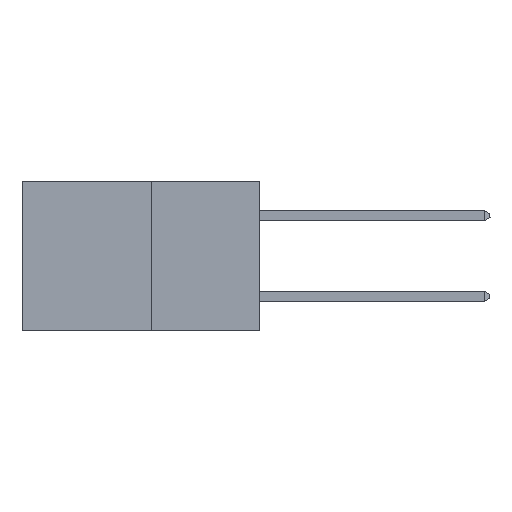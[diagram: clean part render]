
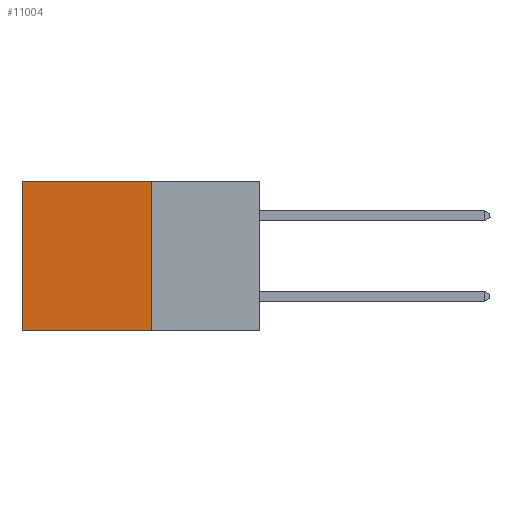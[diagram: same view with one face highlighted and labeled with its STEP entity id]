
A CAD part, left-side view. The second image highlights one B-rep face of the part: STEP entity #11004.
In plain terms, the highlighted planar face has unit normal (-1, 0, 0).
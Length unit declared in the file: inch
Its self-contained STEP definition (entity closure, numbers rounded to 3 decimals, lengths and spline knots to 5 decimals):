
#146 = FACE_OUTER_BOUND ( 'NONE', #1219, .T. ) ;
#1219 = EDGE_LOOP ( 'NONE', ( #10099, #11116, #4568, #2915 ) ) ;
#1784 = DIRECTION ( 'NONE',  ( 0., 1., 0. ) ) ;
#2915 = ORIENTED_EDGE ( 'NONE', *, *, #9272, .T. ) ;
#2984 = LINE ( 'NONE', #14769, #10067 ) ;
#4271 = DIRECTION ( 'NONE',  ( 0., 0., -1. ) ) ;
#4323 = CARTESIAN_POINT ( 'NONE',  ( 0.277, 0.59, -0.37 ) ) ;
#4568 = ORIENTED_EDGE ( 'NONE', *, *, #6917, .F. ) ;
#5737 = EDGE_CURVE ( 'NONE', #11040, #17031, #18094, .T. ) ;
#6049 = CARTESIAN_POINT ( 'NONE',  ( 0.277, 0.59, -0.37 ) ) ;
#6917 = EDGE_CURVE ( 'NONE', #9844, #12047, #13390, .T. ) ;
#6955 = VECTOR ( 'NONE', #4271, 39.37008 ) ;
#8915 = DIRECTION ( 'NONE',  ( 0., 0., -1. ) ) ;
#8993 = CARTESIAN_POINT ( 'NONE',  ( 0.277, 0.27, -0.37 ) ) ;
#9272 = EDGE_CURVE ( 'NONE', #9844, #11040, #13121, .T. ) ;
#9724 = DIRECTION ( 'NONE',  ( 0., 0., -1. ) ) ;
#9748 = VECTOR ( 'NONE', #1784, 39.37008 ) ;
#9844 = VERTEX_POINT ( 'NONE', #9949 ) ;
#9949 = CARTESIAN_POINT ( 'NONE',  ( 0.277, 0.27, 0. ) ) ;
#10067 = VECTOR ( 'NONE', #16122, 39.37008 ) ;
#10099 = ORIENTED_EDGE ( 'NONE', *, *, #5737, .T. ) ;
#10284 = CARTESIAN_POINT ( 'NONE',  ( 0.277, 0.27, 0. ) ) ;
#11004 = ADVANCED_FACE ( 'NONE', ( #146 ), #16634, .F. ) ;
#11040 = VERTEX_POINT ( 'NONE', #11175 ) ;
#11116 = ORIENTED_EDGE ( 'NONE', *, *, #15195, .F. ) ;
#11175 = CARTESIAN_POINT ( 'NONE',  ( 0.277, 0.59, 0. ) ) ;
#11323 = CARTESIAN_POINT ( 'NONE',  ( 0.277, 0.27, -0.37 ) ) ;
#12047 = VERTEX_POINT ( 'NONE', #11323 ) ;
#12934 = VECTOR ( 'NONE', #8915, 39.37008 ) ;
#13121 = LINE ( 'NONE', #10284, #9748 ) ;
#13390 = LINE ( 'NONE', #8993, #12934 ) ;
#13400 = AXIS2_PLACEMENT_3D ( 'NONE', #16684, #18045, #9724 ) ;
#14769 = CARTESIAN_POINT ( 'NONE',  ( 0.277, 0.27, -0.37 ) ) ;
#15195 = EDGE_CURVE ( 'NONE', #12047, #17031, #2984, .T. ) ;
#16122 = DIRECTION ( 'NONE',  ( 0., 1., 0. ) ) ;
#16634 = PLANE ( 'NONE',  #13400 ) ;
#16684 = CARTESIAN_POINT ( 'NONE',  ( 0.277, 0.27, -0.37 ) ) ;
#17031 = VERTEX_POINT ( 'NONE', #6049 ) ;
#18045 = DIRECTION ( 'NONE',  ( 1., 0., 0. ) ) ;
#18094 = LINE ( 'NONE', #4323, #6955 ) ;
